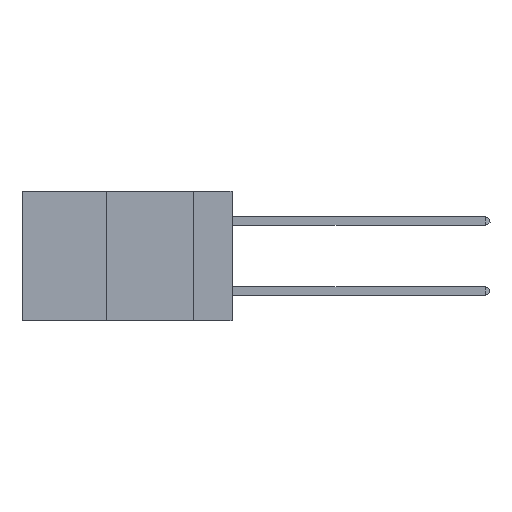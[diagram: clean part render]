
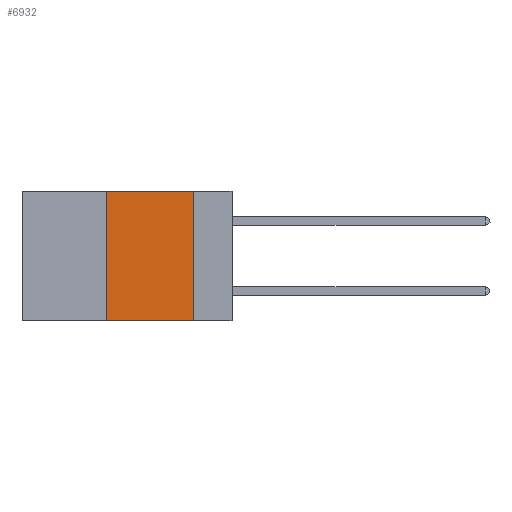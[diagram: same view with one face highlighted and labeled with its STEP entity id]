
A CAD part, left-side view. The second image highlights one B-rep face of the part: STEP entity #6932.
In plain terms, the highlighted planar face has unit normal (-1, 0, 0).
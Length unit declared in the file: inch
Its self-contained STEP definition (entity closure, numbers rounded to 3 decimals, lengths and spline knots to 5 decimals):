
#115 = VECTOR ( 'NONE', #663, 39.37008 ) ;
#663 = DIRECTION ( 'NONE',  ( 0., 0., -1. ) ) ;
#756 = CARTESIAN_POINT ( 'NONE',  ( 0., 0.11, -0.37 ) ) ;
#2063 = ORIENTED_EDGE ( 'NONE', *, *, #11033, .F. ) ;
#2154 = VECTOR ( 'NONE', #6472, 39.37008 ) ;
#2220 = LINE ( 'NONE', #15382, #115 ) ;
#2260 = VECTOR ( 'NONE', #10121, 39.37008 ) ;
#2262 = DIRECTION ( 'NONE',  ( 0., 0., -1. ) ) ;
#2356 = CARTESIAN_POINT ( 'NONE',  ( 0., 0.6, 0. ) ) ;
#2775 = CARTESIAN_POINT ( 'NONE',  ( 0., 0.6, -0.37 ) ) ;
#2907 = EDGE_CURVE ( 'NONE', #5050, #10613, #2220, .T. ) ;
#3869 = VERTEX_POINT ( 'NONE', #13785 ) ;
#4161 = AXIS2_PLACEMENT_3D ( 'NONE', #8385, #9627, #2262 ) ;
#4408 = EDGE_LOOP ( 'NONE', ( #13137, #14844, #2063, #4875 ) ) ;
#4875 = ORIENTED_EDGE ( 'NONE', *, *, #15402, .T. ) ;
#5050 = VERTEX_POINT ( 'NONE', #6272 ) ;
#5402 = LINE ( 'NONE', #2775, #2154 ) ;
#6272 = CARTESIAN_POINT ( 'NONE',  ( 0., 0.11, 0. ) ) ;
#6472 = DIRECTION ( 'NONE',  ( 0., -1., 0. ) ) ;
#6932 = ADVANCED_FACE ( 'NONE', ( #9670 ), #13263, .F. ) ;
#7707 = CARTESIAN_POINT ( 'NONE',  ( 0., 0.36, 0. ) ) ;
#8385 = CARTESIAN_POINT ( 'NONE',  ( 0., 0.6, 0. ) ) ;
#8808 = EDGE_CURVE ( 'NONE', #3869, #5050, #9784, .T. ) ;
#9627 = DIRECTION ( 'NONE',  ( 1., 0., 0. ) ) ;
#9670 = FACE_OUTER_BOUND ( 'NONE', #4408, .T. ) ;
#9784 = LINE ( 'NONE', #2356, #12662 ) ;
#10121 = DIRECTION ( 'NONE',  ( 0., 0., 1. ) ) ;
#10613 = VERTEX_POINT ( 'NONE', #756 ) ;
#11033 = EDGE_CURVE ( 'NONE', #11884, #3869, #13390, .T. ) ;
#11870 = CARTESIAN_POINT ( 'NONE',  ( 0., 0.36, -0.37 ) ) ;
#11884 = VERTEX_POINT ( 'NONE', #11870 ) ;
#12662 = VECTOR ( 'NONE', #14606, 39.37008 ) ;
#13137 = ORIENTED_EDGE ( 'NONE', *, *, #2907, .F. ) ;
#13263 = PLANE ( 'NONE',  #4161 ) ;
#13390 = LINE ( 'NONE', #7707, #2260 ) ;
#13785 = CARTESIAN_POINT ( 'NONE',  ( 0., 0.36, 0. ) ) ;
#14606 = DIRECTION ( 'NONE',  ( 0., -1., 0. ) ) ;
#14844 = ORIENTED_EDGE ( 'NONE', *, *, #8808, .F. ) ;
#15382 = CARTESIAN_POINT ( 'NONE',  ( 0., 0.11, 0. ) ) ;
#15402 = EDGE_CURVE ( 'NONE', #11884, #10613, #5402, .T. ) ;
